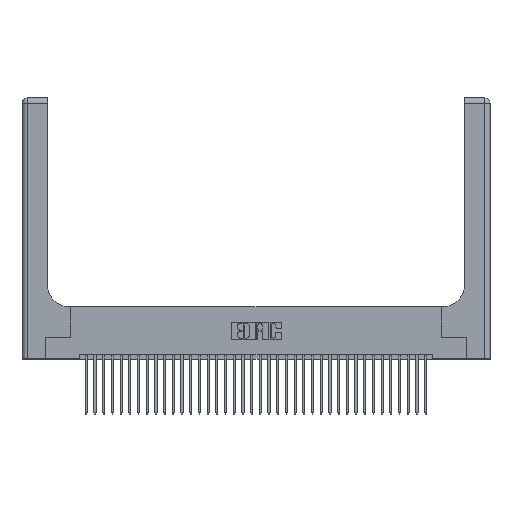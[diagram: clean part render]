
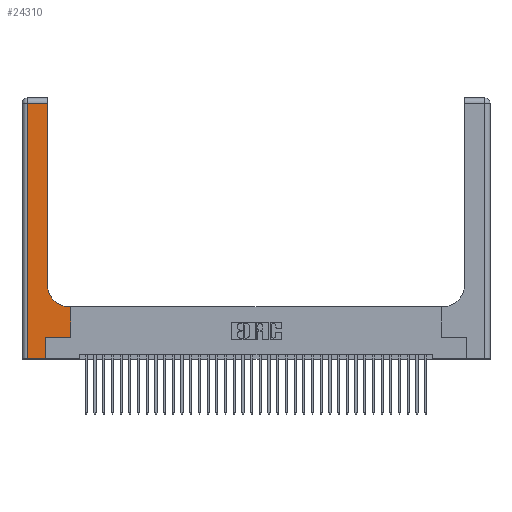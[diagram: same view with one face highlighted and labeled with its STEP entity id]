
A CAD part, top view. The second image highlights one B-rep face of the part: STEP entity #24310.
In plain terms, the highlighted planar face has unit normal (0, 0, 1).
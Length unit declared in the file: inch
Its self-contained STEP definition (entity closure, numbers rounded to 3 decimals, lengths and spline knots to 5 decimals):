
#129 = VECTOR ( 'NONE', #10074, 39.37008 ) ;
#913 = CARTESIAN_POINT ( 'NONE',  ( 0.06, 2.94, 0.37 ) ) ;
#1261 = DIRECTION ( 'NONE',  ( 1., 0., 0. ) ) ;
#1666 = ORIENTED_EDGE ( 'NONE', *, *, #24591, .T. ) ;
#2134 = CARTESIAN_POINT ( 'NONE',  ( 0.2915, 3., 0.37 ) ) ;
#2735 = DIRECTION ( 'NONE',  ( 0., 1., 0. ) ) ;
#2890 = EDGE_CURVE ( 'NONE', #17821, #10076, #15053, .T. ) ;
#3245 = LINE ( 'NONE', #20733, #29932 ) ;
#3413 = ORIENTED_EDGE ( 'NONE', *, *, #9123, .T. ) ;
#3485 = VERTEX_POINT ( 'NONE', #33461 ) ;
#3580 = EDGE_CURVE ( 'NONE', #3485, #10426, #14314, .T. ) ;
#4338 = CARTESIAN_POINT ( 'NONE',  ( 0.5415, 0.85, 0.37 ) ) ;
#4853 = DIRECTION ( 'NONE',  ( 0., -1., 0. ) ) ;
#6816 = AXIS2_PLACEMENT_3D ( 'NONE', #9493, #35090, #31889 ) ;
#7218 = LINE ( 'NONE', #17676, #36668 ) ;
#7420 = CARTESIAN_POINT ( 'NONE',  ( 0.269, 0., 0.37 ) ) ;
#8448 = VECTOR ( 'NONE', #16011, 39.37008 ) ;
#9123 = EDGE_CURVE ( 'NONE', #9470, #3485, #29388, .T. ) ;
#9470 = VERTEX_POINT ( 'NONE', #36007 ) ;
#9493 = CARTESIAN_POINT ( 'NONE',  ( 0., 3., 0.37 ) ) ;
#9834 = EDGE_LOOP ( 'NONE', ( #1666, #27098, #35782, #24818, #15981, #3413, #35791, #34162, #33446 ) ) ;
#10074 = DIRECTION ( 'NONE',  ( -1., 0., 0. ) ) ;
#10076 = VERTEX_POINT ( 'NONE', #28426 ) ;
#10261 = VECTOR ( 'NONE', #14076, 39.37008 ) ;
#10426 = VERTEX_POINT ( 'NONE', #10508 ) ;
#10508 = CARTESIAN_POINT ( 'NONE',  ( 0.5585, 0.6, 0.37 ) ) ;
#10611 = LINE ( 'NONE', #7420, #8448 ) ;
#10716 = CARTESIAN_POINT ( 'NONE',  ( 0.5415, 0.6, 0.37 ) ) ;
#10787 = EDGE_CURVE ( 'NONE', #30943, #9470, #10611, .T. ) ;
#10934 = FACE_OUTER_BOUND ( 'NONE', #9834, .T. ) ;
#12938 = CARTESIAN_POINT ( 'NONE',  ( 0.06, 3., 0.37 ) ) ;
#13345 = DIRECTION ( 'NONE',  ( 0., 1., 0. ) ) ;
#14017 = VERTEX_POINT ( 'NONE', #14791 ) ;
#14051 = VERTEX_POINT ( 'NONE', #10716 ) ;
#14076 = DIRECTION ( 'NONE',  ( 1., 0., 0. ) ) ;
#14314 = LINE ( 'NONE', #16829, #27667 ) ;
#14791 = CARTESIAN_POINT ( 'NONE',  ( 0.2915, 2.94, 0.37 ) ) ;
#15053 = LINE ( 'NONE', #12938, #20802 ) ;
#15981 = ORIENTED_EDGE ( 'NONE', *, *, #10787, .T. ) ;
#16011 = DIRECTION ( 'NONE',  ( 0., 1., 0. ) ) ;
#16829 = CARTESIAN_POINT ( 'NONE',  ( 0.5585, 0.25, 0.37 ) ) ;
#17676 = CARTESIAN_POINT ( 'NONE',  ( 0.2915, 0.6, 0.37 ) ) ;
#17812 = PLANE ( 'NONE',  #6816 ) ;
#17821 = VERTEX_POINT ( 'NONE', #913 ) ;
#19275 = EDGE_CURVE ( 'NONE', #10426, #14051, #7218, .T. ) ;
#19344 = EDGE_CURVE ( 'NONE', #14051, #22121, #35216, .T. ) ;
#20635 = VECTOR ( 'NONE', #13345, 39.37008 ) ;
#20733 = CARTESIAN_POINT ( 'NONE',  ( 0., 0., 0.37 ) ) ;
#20802 = VECTOR ( 'NONE', #4853, 39.37008 ) ;
#20988 = CARTESIAN_POINT ( 'NONE',  ( 0.2915, 0.85, 0.37 ) ) ;
#21254 = CARTESIAN_POINT ( 'NONE',  ( 0., 2.94, 0.37 ) ) ;
#21261 = DIRECTION ( 'NONE',  ( 0., 0., -1. ) ) ;
#22121 = VERTEX_POINT ( 'NONE', #20988 ) ;
#22389 = CARTESIAN_POINT ( 'NONE',  ( 0.269, 0.25, 0.37 ) ) ;
#24310 = ADVANCED_FACE ( 'NONE', ( #10934 ), #17812, .F. ) ;
#24591 = EDGE_CURVE ( 'NONE', #22121, #14017, #28320, .T. ) ;
#24818 = ORIENTED_EDGE ( 'NONE', *, *, #30525, .T. ) ;
#24951 = DIRECTION ( 'NONE',  ( -1., 0., 0. ) ) ;
#27098 = ORIENTED_EDGE ( 'NONE', *, *, #36473, .T. ) ;
#27667 = VECTOR ( 'NONE', #2735, 39.37008 ) ;
#28161 = CARTESIAN_POINT ( 'NONE',  ( 0.269, 0., 0.37 ) ) ;
#28320 = LINE ( 'NONE', #2134, #20635 ) ;
#28426 = CARTESIAN_POINT ( 'NONE',  ( 0.06, 0., 0.37 ) ) ;
#29388 = LINE ( 'NONE', #22389, #10261 ) ;
#29932 = VECTOR ( 'NONE', #35143, 39.37008 ) ;
#30525 = EDGE_CURVE ( 'NONE', #10076, #30943, #3245, .T. ) ;
#30943 = VERTEX_POINT ( 'NONE', #28161 ) ;
#31344 = LINE ( 'NONE', #21254, #129 ) ;
#31889 = DIRECTION ( 'NONE',  ( -1., 0., 0. ) ) ;
#33446 = ORIENTED_EDGE ( 'NONE', *, *, #19344, .T. ) ;
#33461 = CARTESIAN_POINT ( 'NONE',  ( 0.5585, 0.25, 0.37 ) ) ;
#34162 = ORIENTED_EDGE ( 'NONE', *, *, #19275, .T. ) ;
#35090 = DIRECTION ( 'NONE',  ( 0., 0., -1. ) ) ;
#35143 = DIRECTION ( 'NONE',  ( 1., 0., 0. ) ) ;
#35216 = CIRCLE ( 'NONE', #35613, 0.25 ) ;
#35613 = AXIS2_PLACEMENT_3D ( 'NONE', #4338, #21261, #1261 ) ;
#35782 = ORIENTED_EDGE ( 'NONE', *, *, #2890, .T. ) ;
#35791 = ORIENTED_EDGE ( 'NONE', *, *, #3580, .T. ) ;
#36007 = CARTESIAN_POINT ( 'NONE',  ( 0.269, 0.25, 0.37 ) ) ;
#36473 = EDGE_CURVE ( 'NONE', #14017, #17821, #31344, .T. ) ;
#36668 = VECTOR ( 'NONE', #24951, 39.37008 ) ;
